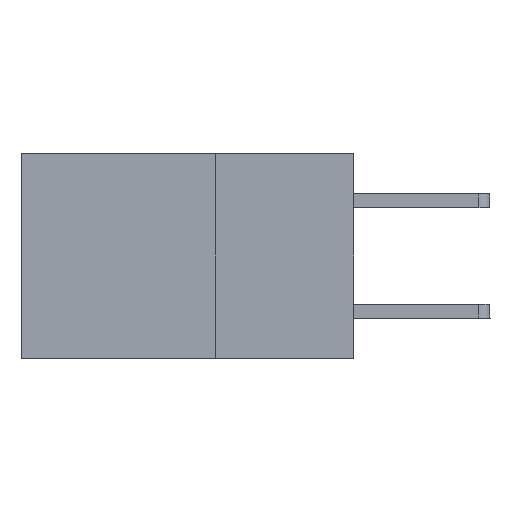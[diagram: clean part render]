
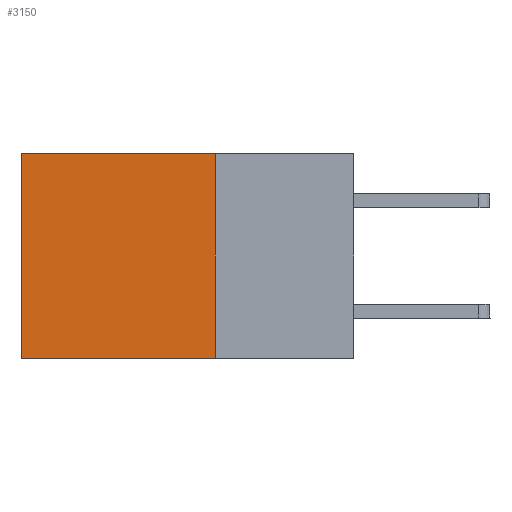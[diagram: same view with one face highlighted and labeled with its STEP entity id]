
A CAD part, left-side view. The second image highlights one B-rep face of the part: STEP entity #3150.
In plain terms, the highlighted planar face has unit normal (-1, 0, 0).
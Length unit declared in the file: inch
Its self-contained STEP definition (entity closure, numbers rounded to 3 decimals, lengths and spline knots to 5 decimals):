
#740 = ORIENTED_EDGE ( 'NONE', *, *, #3600, .F. ) ;
#814 = LINE ( 'NONE', #2568, #9525 ) ;
#858 = CARTESIAN_POINT ( 'NONE',  ( 0.2875, 0.25, 0. ) ) ;
#1475 = ORIENTED_EDGE ( 'NONE', *, *, #7628, .T. ) ;
#1688 = AXIS2_PLACEMENT_3D ( 'NONE', #11378, #9414, #12092 ) ;
#1765 = DIRECTION ( 'NONE',  ( 0., 0., -1. ) ) ;
#2292 = VERTEX_POINT ( 'NONE', #5556 ) ;
#2568 = CARTESIAN_POINT ( 'NONE',  ( 0.2875, 0.25, -0.37 ) ) ;
#2748 = LINE ( 'NONE', #10610, #5102 ) ;
#2870 = VERTEX_POINT ( 'NONE', #11010 ) ;
#3150 = ADVANCED_FACE ( 'NONE', ( #3409 ), #5337, .F. ) ;
#3409 = FACE_OUTER_BOUND ( 'NONE', #5449, .T. ) ;
#3528 = EDGE_CURVE ( 'NONE', #2292, #7811, #7378, .T. ) ;
#3600 = EDGE_CURVE ( 'NONE', #2870, #7811, #814, .T. ) ;
#3869 = ORIENTED_EDGE ( 'NONE', *, *, #3528, .T. ) ;
#4281 = VERTEX_POINT ( 'NONE', #7443 ) ;
#4782 = LINE ( 'NONE', #858, #8398 ) ;
#5102 = VECTOR ( 'NONE', #1765, 39.37008 ) ;
#5337 = PLANE ( 'NONE',  #1688 ) ;
#5449 = EDGE_LOOP ( 'NONE', ( #3869, #740, #10201, #1475 ) ) ;
#5556 = CARTESIAN_POINT ( 'NONE',  ( 0.2875, 0.6, 0. ) ) ;
#7201 = EDGE_CURVE ( 'NONE', #4281, #2870, #2748, .T. ) ;
#7378 = LINE ( 'NONE', #12297, #12610 ) ;
#7441 = DIRECTION ( 'NONE',  ( 0., 0., -1. ) ) ;
#7443 = CARTESIAN_POINT ( 'NONE',  ( 0.2875, 0.25, 0. ) ) ;
#7628 = EDGE_CURVE ( 'NONE', #4281, #2292, #4782, .T. ) ;
#7811 = VERTEX_POINT ( 'NONE', #8607 ) ;
#8398 = VECTOR ( 'NONE', #8710, 39.37008 ) ;
#8607 = CARTESIAN_POINT ( 'NONE',  ( 0.2875, 0.6, -0.37 ) ) ;
#8710 = DIRECTION ( 'NONE',  ( 0., 1., 0. ) ) ;
#9414 = DIRECTION ( 'NONE',  ( 1., 0., 0. ) ) ;
#9525 = VECTOR ( 'NONE', #12617, 39.37008 ) ;
#10201 = ORIENTED_EDGE ( 'NONE', *, *, #7201, .F. ) ;
#10610 = CARTESIAN_POINT ( 'NONE',  ( 0.2875, 0.25, 0. ) ) ;
#11010 = CARTESIAN_POINT ( 'NONE',  ( 0.2875, 0.25, -0.37 ) ) ;
#11378 = CARTESIAN_POINT ( 'NONE',  ( 0.2875, 0.25, 0. ) ) ;
#12092 = DIRECTION ( 'NONE',  ( 0., 0., -1. ) ) ;
#12297 = CARTESIAN_POINT ( 'NONE',  ( 0.2875, 0.6, 0. ) ) ;
#12610 = VECTOR ( 'NONE', #7441, 39.37008 ) ;
#12617 = DIRECTION ( 'NONE',  ( 0., 1., 0. ) ) ;
